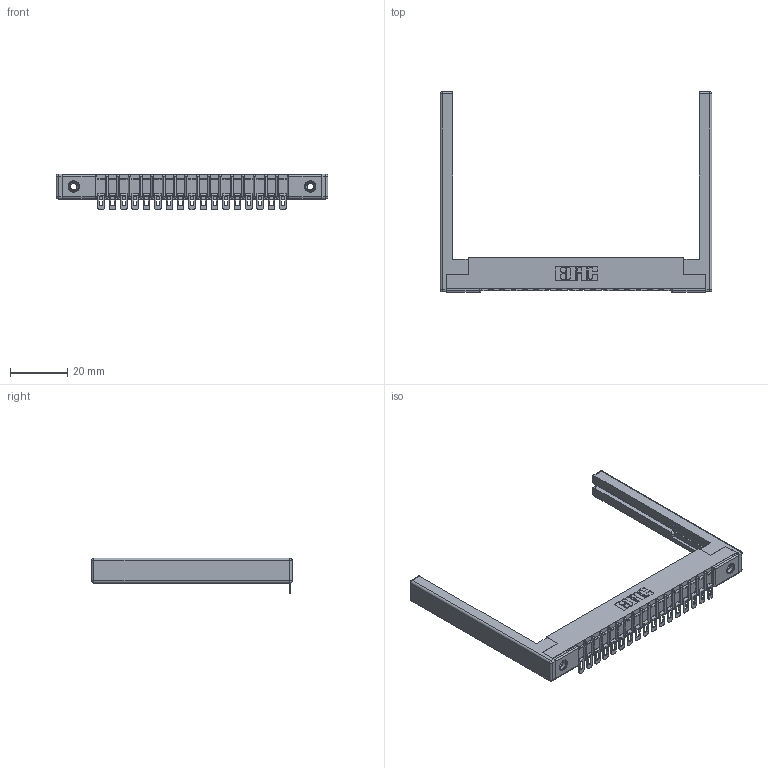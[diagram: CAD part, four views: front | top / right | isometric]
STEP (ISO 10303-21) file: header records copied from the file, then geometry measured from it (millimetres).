
FILE_DESCRIPTION (( 'STEP AP203' ), '1' );
FILE_NAME ('307-017-554-168.STEP', '2019-09-04T21:57:40', ( '' ), ( '' ), 'SwSTEP 2.0', 'SolidWorks 2016', '' );
FILE_SCHEMA (( 'CONFIG_CONTROL_DESIGN' ));
Length unit declared in the file: inch
Products named in the file (5): 307 Part_.156 Dia Mounting Holes; 345-250-001_345-250-001-102; 307-017-554-168; 307-220-068; 307-290-002_554
Assembly tree (22 placements, depth 2):
  307-017-554-168
    307 Part_.156 Dia Mounting Holes
    307-290-002_554  x17
    307-220-068  x2
    345-250-001_345-250-001-102  x2
Bounding box: 94.79 x 69.98 x 12.52 mm (x, y, z)
Volume: 10820.3 mm3; surface area: 15201.2 mm2
Topology: 22 solids, 22 shells, 1667 faces, 5014 edges, 3272 vertices
Faces by surface type: plane 940, cylinder 667, sphere 44, cone 12, torus 4
Entity records: 21380 total; most frequent: CARTESIAN_POINT 3567, ORIENTED_EDGE 3546, DIRECTION 3501, EDGE_CURVE 1773, VECTOR 1337, LINE 1337, VERTEX_POINT 1148, AXIS2_PLACEMENT_3D 1082
